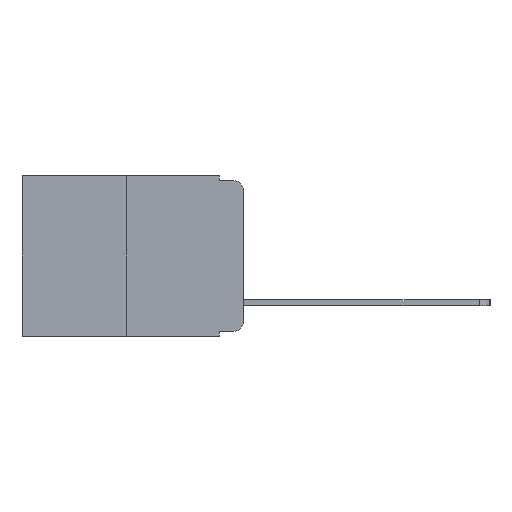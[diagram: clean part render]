
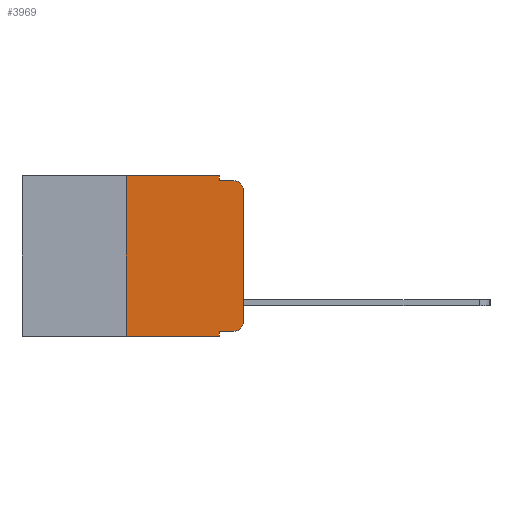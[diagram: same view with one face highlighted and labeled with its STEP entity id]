
A CAD part, left-side view. The second image highlights one B-rep face of the part: STEP entity #3969.
In plain terms, the highlighted planar face has unit normal (-1, 0, 0).
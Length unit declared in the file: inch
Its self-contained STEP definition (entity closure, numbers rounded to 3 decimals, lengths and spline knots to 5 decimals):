
#333 = DIRECTION ( 'NONE',  ( 0., 0., -1. ) ) ;
#491 = CARTESIAN_POINT ( 'NONE',  ( 0., 0.02, -0.333 ) ) ;
#844 = CARTESIAN_POINT ( 'NONE',  ( 0., 0.02, -0.313 ) ) ;
#1089 = EDGE_CURVE ( 'NONE', #22323, #15507, #13741, .T. ) ;
#1727 = VECTOR ( 'NONE', #17678, 39.37008 ) ;
#2329 = VERTEX_POINT ( 'NONE', #19518 ) ;
#2843 = AXIS2_PLACEMENT_3D ( 'NONE', #844, #11125, #4822 ) ;
#3195 = ORIENTED_EDGE ( 'NONE', *, *, #11214, .T. ) ;
#3552 = LINE ( 'NONE', #23386, #12832 ) ;
#3969 = ADVANCED_FACE ( 'NONE', ( #22409 ), #22334, .F. ) ;
#4306 = VERTEX_POINT ( 'NONE', #20622 ) ;
#4822 = DIRECTION ( 'NONE',  ( 0., 0., -1. ) ) ;
#5008 = EDGE_CURVE ( 'NONE', #16612, #22323, #22080, .T. ) ;
#5425 = CARTESIAN_POINT ( 'NONE',  ( 0., 0.051, -0.333 ) ) ;
#6284 = EDGE_CURVE ( 'NONE', #16612, #9716, #20604, .T. ) ;
#6716 = CARTESIAN_POINT ( 'NONE',  ( 0., 0.25, -0.343 ) ) ;
#6729 = VECTOR ( 'NONE', #19415, 39.37008 ) ;
#7193 = VECTOR ( 'NONE', #18597, 39.37008 ) ;
#7415 = LINE ( 'NONE', #15962, #1727 ) ;
#7525 = EDGE_CURVE ( 'NONE', #17649, #9402, #19471, .T. ) ;
#7632 = VERTEX_POINT ( 'NONE', #17532 ) ;
#8079 = CARTESIAN_POINT ( 'NONE',  ( 0., 0.473, 0. ) ) ;
#8206 = ORIENTED_EDGE ( 'NONE', *, *, #10018, .F. ) ;
#8271 = CARTESIAN_POINT ( 'NONE',  ( 0., 0.25, 0. ) ) ;
#8767 = EDGE_CURVE ( 'NONE', #7632, #4306, #7415, .T. ) ;
#8921 = LINE ( 'NONE', #9759, #7193 ) ;
#8955 = AXIS2_PLACEMENT_3D ( 'NONE', #21281, #10737, #23089 ) ;
#9376 = ORIENTED_EDGE ( 'NONE', *, *, #12272, .F. ) ;
#9402 = VERTEX_POINT ( 'NONE', #23258 ) ;
#9417 = EDGE_LOOP ( 'NONE', ( #17208, #3195, #8206, #18275, #9376, #9970, #10551, #19912, #16421, #12791 ) ) ;
#9503 = VECTOR ( 'NONE', #18941, 39.37008 ) ;
#9716 = VERTEX_POINT ( 'NONE', #20433 ) ;
#9759 = CARTESIAN_POINT ( 'NONE',  ( 0., 0.473, -0.343 ) ) ;
#9970 = ORIENTED_EDGE ( 'NONE', *, *, #7525, .F. ) ;
#10018 = EDGE_CURVE ( 'NONE', #4306, #2329, #3552, .T. ) ;
#10202 = VECTOR ( 'NONE', #15335, 39.37008 ) ;
#10472 = DIRECTION ( 'NONE',  ( 1., 0., 0. ) ) ;
#10551 = ORIENTED_EDGE ( 'NONE', *, *, #15600, .T. ) ;
#10737 = DIRECTION ( 'NONE',  ( -1., 0., 0. ) ) ;
#11000 = CARTESIAN_POINT ( 'NONE',  ( 0., 0.051, -0.333 ) ) ;
#11125 = DIRECTION ( 'NONE',  ( -1., 0., 0. ) ) ;
#11214 = EDGE_CURVE ( 'NONE', #23199, #2329, #17204, .T. ) ;
#11224 = VECTOR ( 'NONE', #333, 39.37008 ) ;
#12272 = EDGE_CURVE ( 'NONE', #9402, #7632, #14403, .T. ) ;
#12418 = EDGE_CURVE ( 'NONE', #15507, #23199, #16356, .T. ) ;
#12731 = DIRECTION ( 'NONE',  ( 0., -1., 0. ) ) ;
#12791 = ORIENTED_EDGE ( 'NONE', *, *, #1089, .T. ) ;
#12832 = VECTOR ( 'NONE', #18140, 39.37008 ) ;
#13531 = CARTESIAN_POINT ( 'NONE',  ( 0., 0.473, 0. ) ) ;
#13741 = CIRCLE ( 'NONE', #2843, 0.02 ) ;
#14403 = LINE ( 'NONE', #13531, #10202 ) ;
#15293 = CARTESIAN_POINT ( 'NONE',  ( 0., 0.051, 0. ) ) ;
#15335 = DIRECTION ( 'NONE',  ( 0., -1., 0. ) ) ;
#15507 = VERTEX_POINT ( 'NONE', #20202 ) ;
#15600 = EDGE_CURVE ( 'NONE', #17649, #9716, #8921, .T. ) ;
#15962 = CARTESIAN_POINT ( 'NONE',  ( 0., 0.051, 0. ) ) ;
#16356 = LINE ( 'NONE', #17687, #6729 ) ;
#16421 = ORIENTED_EDGE ( 'NONE', *, *, #5008, .T. ) ;
#16612 = VERTEX_POINT ( 'NONE', #11000 ) ;
#17204 = CIRCLE ( 'NONE', #8955, 0.02 ) ;
#17208 = ORIENTED_EDGE ( 'NONE', *, *, #12418, .T. ) ;
#17425 = VECTOR ( 'NONE', #12731, 39.37008 ) ;
#17532 = CARTESIAN_POINT ( 'NONE',  ( 0., 0.051, 0. ) ) ;
#17536 = DIRECTION ( 'NONE',  ( 0., 0., -1. ) ) ;
#17649 = VERTEX_POINT ( 'NONE', #6716 ) ;
#17678 = DIRECTION ( 'NONE',  ( 0., 0., -1. ) ) ;
#17687 = CARTESIAN_POINT ( 'NONE',  ( 0., 0., 0. ) ) ;
#18140 = DIRECTION ( 'NONE',  ( 0., -1., 0. ) ) ;
#18275 = ORIENTED_EDGE ( 'NONE', *, *, #8767, .F. ) ;
#18597 = DIRECTION ( 'NONE',  ( 0., -1., 0. ) ) ;
#18941 = DIRECTION ( 'NONE',  ( 0., 0., 1. ) ) ;
#19415 = DIRECTION ( 'NONE',  ( 0., 0., 1. ) ) ;
#19471 = LINE ( 'NONE', #8271, #9503 ) ;
#19518 = CARTESIAN_POINT ( 'NONE',  ( 0., 0.02, -0.01 ) ) ;
#19770 = CARTESIAN_POINT ( 'NONE',  ( 0., 0., -0.03 ) ) ;
#19912 = ORIENTED_EDGE ( 'NONE', *, *, #6284, .F. ) ;
#20202 = CARTESIAN_POINT ( 'NONE',  ( 0., 0., -0.313 ) ) ;
#20433 = CARTESIAN_POINT ( 'NONE',  ( 0., 0.051, -0.343 ) ) ;
#20604 = LINE ( 'NONE', #15293, #11224 ) ;
#20622 = CARTESIAN_POINT ( 'NONE',  ( 0., 0.051, -0.01 ) ) ;
#21281 = CARTESIAN_POINT ( 'NONE',  ( 0., 0.02, -0.03 ) ) ;
#22080 = LINE ( 'NONE', #5425, #17425 ) ;
#22134 = AXIS2_PLACEMENT_3D ( 'NONE', #8079, #10472, #17536 ) ;
#22323 = VERTEX_POINT ( 'NONE', #491 ) ;
#22334 = PLANE ( 'NONE',  #22134 ) ;
#22409 = FACE_OUTER_BOUND ( 'NONE', #9417, .T. ) ;
#23089 = DIRECTION ( 'NONE',  ( 0., 0., -1. ) ) ;
#23199 = VERTEX_POINT ( 'NONE', #19770 ) ;
#23258 = CARTESIAN_POINT ( 'NONE',  ( 0., 0.25, 0. ) ) ;
#23386 = CARTESIAN_POINT ( 'NONE',  ( 0., 0.051, -0.01 ) ) ;
